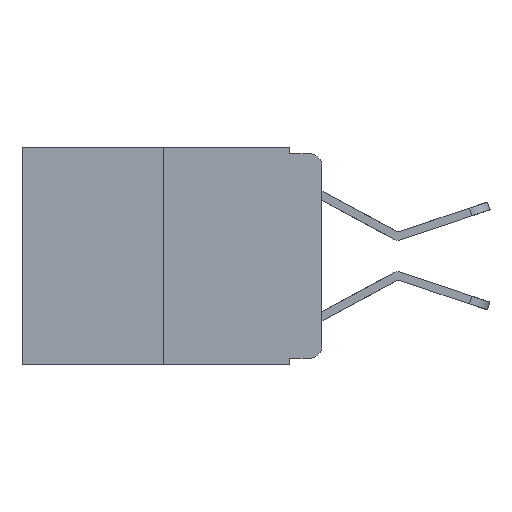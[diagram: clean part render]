
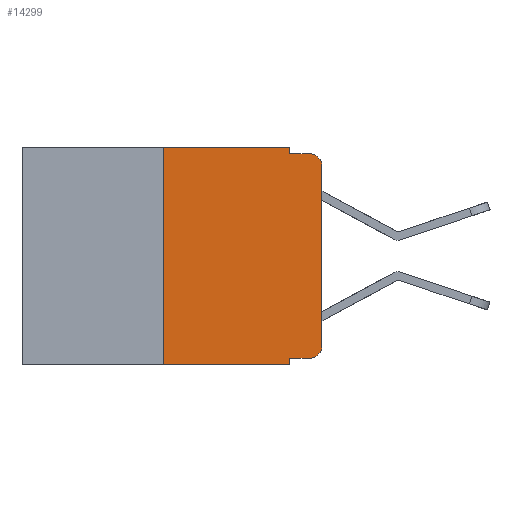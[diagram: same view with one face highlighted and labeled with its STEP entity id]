
A CAD part, left-side view. The second image highlights one B-rep face of the part: STEP entity #14299.
In plain terms, the highlighted planar face has unit normal (-1, 0, 0).
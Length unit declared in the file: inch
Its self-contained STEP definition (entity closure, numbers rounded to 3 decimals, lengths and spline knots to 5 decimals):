
#287 = CARTESIAN_POINT ( 'NONE',  ( 0., 0.473, 0. ) ) ;
#323 = ORIENTED_EDGE ( 'NONE', *, *, #13033, .T. ) ;
#648 = DIRECTION ( 'NONE',  ( -1., 0., 0. ) ) ;
#683 = EDGE_CURVE ( 'NONE', #17490, #8150, #14397, .T. ) ;
#687 = CARTESIAN_POINT ( 'NONE',  ( 0., 0.473, -0.343 ) ) ;
#727 = CARTESIAN_POINT ( 'NONE',  ( 0., 0.02, -0.03 ) ) ;
#936 = ORIENTED_EDGE ( 'NONE', *, *, #16117, .F. ) ;
#1004 = VECTOR ( 'NONE', #14189, 39.37008 ) ;
#1125 = VERTEX_POINT ( 'NONE', #19060 ) ;
#1573 = CARTESIAN_POINT ( 'NONE',  ( 0., 0.25, -0.343 ) ) ;
#1593 = ORIENTED_EDGE ( 'NONE', *, *, #683, .F. ) ;
#1870 = EDGE_CURVE ( 'NONE', #8150, #5295, #15078, .T. ) ;
#2276 = CARTESIAN_POINT ( 'NONE',  ( 0., 0., -0.313 ) ) ;
#2541 = LINE ( 'NONE', #15259, #16158 ) ;
#2840 = EDGE_CURVE ( 'NONE', #14996, #17490, #5987, .T. ) ;
#2897 = VECTOR ( 'NONE', #6793, 39.37008 ) ;
#3135 = ORIENTED_EDGE ( 'NONE', *, *, #10944, .T. ) ;
#3546 = CARTESIAN_POINT ( 'NONE',  ( 0., 0.051, -0.343 ) ) ;
#3783 = DIRECTION ( 'NONE',  ( 1., 0., 0. ) ) ;
#4118 = EDGE_CURVE ( 'NONE', #13942, #5295, #20254, .T. ) ;
#5295 = VERTEX_POINT ( 'NONE', #13215 ) ;
#5708 = ORIENTED_EDGE ( 'NONE', *, *, #8313, .T. ) ;
#5768 = ORIENTED_EDGE ( 'NONE', *, *, #14070, .F. ) ;
#5987 = LINE ( 'NONE', #287, #10707 ) ;
#6793 = DIRECTION ( 'NONE',  ( 0., -1., 0. ) ) ;
#7021 = LINE ( 'NONE', #9771, #19386 ) ;
#7058 = AXIS2_PLACEMENT_3D ( 'NONE', #727, #648, #10095 ) ;
#7383 = EDGE_CURVE ( 'NONE', #15480, #13942, #8739, .T. ) ;
#7527 = ORIENTED_EDGE ( 'NONE', *, *, #2840, .F. ) ;
#7605 = FACE_OUTER_BOUND ( 'NONE', #14519, .T. ) ;
#7647 = DIRECTION ( 'NONE',  ( -1., 0., 0. ) ) ;
#7656 = CARTESIAN_POINT ( 'NONE',  ( 0., 0.051, -0.01 ) ) ;
#8044 = DIRECTION ( 'NONE',  ( 0., 0., -1. ) ) ;
#8150 = VERTEX_POINT ( 'NONE', #16312 ) ;
#8313 = EDGE_CURVE ( 'NONE', #10869, #10013, #20504, .T. ) ;
#8324 = ORIENTED_EDGE ( 'NONE', *, *, #1870, .F. ) ;
#8739 = LINE ( 'NONE', #12641, #1004 ) ;
#9228 = ORIENTED_EDGE ( 'NONE', *, *, #4118, .T. ) ;
#9768 = VECTOR ( 'NONE', #8044, 39.37008 ) ;
#9771 = CARTESIAN_POINT ( 'NONE',  ( 0., 0.25, 0. ) ) ;
#9896 = CARTESIAN_POINT ( 'NONE',  ( 0., 0.02, -0.313 ) ) ;
#9924 = AXIS2_PLACEMENT_3D ( 'NONE', #9896, #7647, #11485 ) ;
#10013 = VERTEX_POINT ( 'NONE', #3546 ) ;
#10095 = DIRECTION ( 'NONE',  ( 0., 0., -1. ) ) ;
#10691 = CARTESIAN_POINT ( 'NONE',  ( 0., 0.25, 0. ) ) ;
#10707 = VECTOR ( 'NONE', #11566, 39.37008 ) ;
#10869 = VERTEX_POINT ( 'NONE', #1573 ) ;
#10944 = EDGE_CURVE ( 'NONE', #13275, #15480, #16134, .T. ) ;
#11485 = DIRECTION ( 'NONE',  ( 0., 0., -1. ) ) ;
#11566 = DIRECTION ( 'NONE',  ( 0., -1., 0. ) ) ;
#12641 = CARTESIAN_POINT ( 'NONE',  ( 0., 0., 0. ) ) ;
#12728 = ORIENTED_EDGE ( 'NONE', *, *, #7383, .T. ) ;
#12761 = CARTESIAN_POINT ( 'NONE',  ( 0., 0.051, 0. ) ) ;
#12865 = VECTOR ( 'NONE', #19724, 39.37008 ) ;
#13033 = EDGE_CURVE ( 'NONE', #1125, #13275, #2541, .T. ) ;
#13215 = CARTESIAN_POINT ( 'NONE',  ( 0., 0.02, -0.01 ) ) ;
#13275 = VERTEX_POINT ( 'NONE', #15415 ) ;
#13311 = CARTESIAN_POINT ( 'NONE',  ( 0., 0.473, 0. ) ) ;
#13942 = VERTEX_POINT ( 'NONE', #17111 ) ;
#14070 = EDGE_CURVE ( 'NONE', #1125, #10013, #15867, .T. ) ;
#14189 = DIRECTION ( 'NONE',  ( 0., 0., 1. ) ) ;
#14299 = ADVANCED_FACE ( 'NONE', ( #7605 ), #19383, .F. ) ;
#14397 = LINE ( 'NONE', #18473, #9768 ) ;
#14402 = DIRECTION ( 'NONE',  ( 0., 0., 1. ) ) ;
#14519 = EDGE_LOOP ( 'NONE', ( #12728, #9228, #8324, #1593, #7527, #936, #5708, #5768, #323, #3135 ) ) ;
#14848 = DIRECTION ( 'NONE',  ( 0., 0., -1. ) ) ;
#14996 = VERTEX_POINT ( 'NONE', #10691 ) ;
#15078 = LINE ( 'NONE', #7656, #2897 ) ;
#15259 = CARTESIAN_POINT ( 'NONE',  ( 0., 0.051, -0.333 ) ) ;
#15415 = CARTESIAN_POINT ( 'NONE',  ( 0., 0.02, -0.333 ) ) ;
#15480 = VERTEX_POINT ( 'NONE', #2276 ) ;
#15867 = LINE ( 'NONE', #12761, #19458 ) ;
#16058 = AXIS2_PLACEMENT_3D ( 'NONE', #13311, #3783, #14848 ) ;
#16117 = EDGE_CURVE ( 'NONE', #10869, #14996, #7021, .T. ) ;
#16134 = CIRCLE ( 'NONE', #9924, 0.02 ) ;
#16158 = VECTOR ( 'NONE', #19803, 39.37008 ) ;
#16312 = CARTESIAN_POINT ( 'NONE',  ( 0., 0.051, -0.01 ) ) ;
#17111 = CARTESIAN_POINT ( 'NONE',  ( 0., 0., -0.03 ) ) ;
#17490 = VERTEX_POINT ( 'NONE', #17760 ) ;
#17760 = CARTESIAN_POINT ( 'NONE',  ( 0., 0.051, 0. ) ) ;
#18473 = CARTESIAN_POINT ( 'NONE',  ( 0., 0.051, 0. ) ) ;
#19060 = CARTESIAN_POINT ( 'NONE',  ( 0., 0.051, -0.333 ) ) ;
#19383 = PLANE ( 'NONE',  #16058 ) ;
#19386 = VECTOR ( 'NONE', #14402, 39.37008 ) ;
#19458 = VECTOR ( 'NONE', #20376, 39.37008 ) ;
#19724 = DIRECTION ( 'NONE',  ( 0., -1., 0. ) ) ;
#19803 = DIRECTION ( 'NONE',  ( 0., -1., 0. ) ) ;
#20254 = CIRCLE ( 'NONE', #7058, 0.02 ) ;
#20376 = DIRECTION ( 'NONE',  ( 0., 0., -1. ) ) ;
#20504 = LINE ( 'NONE', #687, #12865 ) ;
